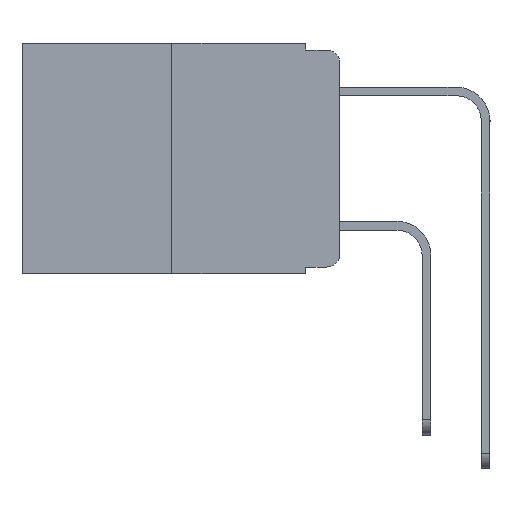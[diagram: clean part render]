
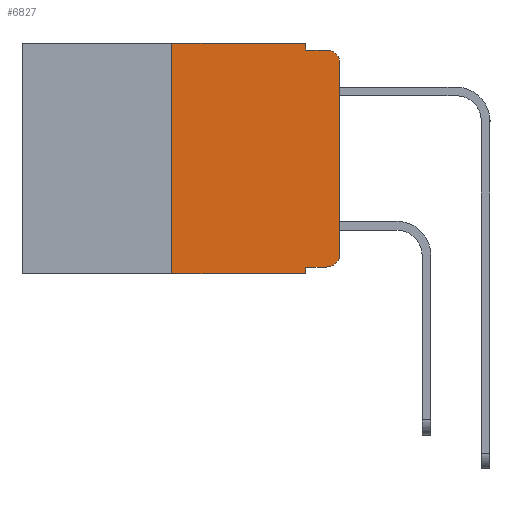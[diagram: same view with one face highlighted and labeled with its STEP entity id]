
A CAD part, left-side view. The second image highlights one B-rep face of the part: STEP entity #6827.
In plain terms, the highlighted planar face has unit normal (-1, 0, 0).
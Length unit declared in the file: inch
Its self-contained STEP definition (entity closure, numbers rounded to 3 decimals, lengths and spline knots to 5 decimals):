
#194 = ORIENTED_EDGE ( 'NONE', *, *, #5802, .T. ) ;
#305 = ORIENTED_EDGE ( 'NONE', *, *, #12336, .F. ) ;
#312 = PLANE ( 'NONE',  #7503 ) ;
#669 = LINE ( 'NONE', #23085, #15810 ) ;
#783 = VECTOR ( 'NONE', #23891, 39.37008 ) ;
#924 = ORIENTED_EDGE ( 'NONE', *, *, #17649, .T. ) ;
#1150 = EDGE_CURVE ( 'NONE', #8690, #19182, #22204, .T. ) ;
#1744 = CARTESIAN_POINT ( 'NONE',  ( 0., 0.051, 0. ) ) ;
#2332 = CARTESIAN_POINT ( 'NONE',  ( 0., 0., -0.313 ) ) ;
#2387 = ORIENTED_EDGE ( 'NONE', *, *, #1150, .F. ) ;
#2409 = VERTEX_POINT ( 'NONE', #2792 ) ;
#2776 = ORIENTED_EDGE ( 'NONE', *, *, #11029, .F. ) ;
#2792 = CARTESIAN_POINT ( 'NONE',  ( 0., 0.051, -0.01 ) ) ;
#3441 = DIRECTION ( 'NONE',  ( -1., 0., 0. ) ) ;
#3478 = DIRECTION ( 'NONE',  ( 0., 0., -1. ) ) ;
#3485 = EDGE_CURVE ( 'NONE', #17814, #13429, #20283, .T. ) ;
#3825 = ORIENTED_EDGE ( 'NONE', *, *, #8395, .F. ) ;
#4026 = CARTESIAN_POINT ( 'NONE',  ( 0., 0.02, -0.333 ) ) ;
#4243 = VERTEX_POINT ( 'NONE', #4026 ) ;
#4704 = CARTESIAN_POINT ( 'NONE',  ( 0., 0.051, -0.343 ) ) ;
#5216 = CARTESIAN_POINT ( 'NONE',  ( 0., 0.02, -0.313 ) ) ;
#5350 = CARTESIAN_POINT ( 'NONE',  ( 0., 0.051, 0. ) ) ;
#5802 = EDGE_CURVE ( 'NONE', #4243, #10560, #9116, .T. ) ;
#6376 = FACE_OUTER_BOUND ( 'NONE', #19559, .T. ) ;
#6600 = VECTOR ( 'NONE', #23822, 39.37008 ) ;
#6827 = ADVANCED_FACE ( 'NONE', ( #6376 ), #312, .F. ) ;
#7114 = EDGE_CURVE ( 'NONE', #15559, #4243, #21062, .T. ) ;
#7503 = AXIS2_PLACEMENT_3D ( 'NONE', #17648, #24567, #24156 ) ;
#7657 = CIRCLE ( 'NONE', #21750, 0.02 ) ;
#7786 = ORIENTED_EDGE ( 'NONE', *, *, #7114, .T. ) ;
#8268 = CARTESIAN_POINT ( 'NONE',  ( 0., 0.051, -0.01 ) ) ;
#8365 = CARTESIAN_POINT ( 'NONE',  ( 0., 0.02, -0.03 ) ) ;
#8395 = EDGE_CURVE ( 'NONE', #15559, #13429, #669, .T. ) ;
#8479 = DIRECTION ( 'NONE',  ( 0., -1., 0. ) ) ;
#8690 = VERTEX_POINT ( 'NONE', #20181 ) ;
#9111 = CARTESIAN_POINT ( 'NONE',  ( 0., 0.473, -0.343 ) ) ;
#9116 = CIRCLE ( 'NONE', #22555, 0.02 ) ;
#9568 = ORIENTED_EDGE ( 'NONE', *, *, #15020, .F. ) ;
#9575 = LINE ( 'NONE', #5350, #14199 ) ;
#9639 = VECTOR ( 'NONE', #15490, 39.37008 ) ;
#9720 = ORIENTED_EDGE ( 'NONE', *, *, #16343, .T. ) ;
#9856 = VECTOR ( 'NONE', #8479, 39.37008 ) ;
#10327 = DIRECTION ( 'NONE',  ( 0., 0., -1. ) ) ;
#10560 = VERTEX_POINT ( 'NONE', #2332 ) ;
#11029 = EDGE_CURVE ( 'NONE', #17814, #8690, #25164, .T. ) ;
#11262 = LINE ( 'NONE', #8268, #783 ) ;
#12336 = EDGE_CURVE ( 'NONE', #19182, #2409, #9575, .T. ) ;
#12668 = CARTESIAN_POINT ( 'NONE',  ( 0., 0.051, -0.333 ) ) ;
#13429 = VERTEX_POINT ( 'NONE', #4704 ) ;
#13446 = CARTESIAN_POINT ( 'NONE',  ( 0., 0.473, 0. ) ) ;
#13503 = CARTESIAN_POINT ( 'NONE',  ( 0., 0.25, 0. ) ) ;
#14199 = VECTOR ( 'NONE', #17154, 39.37008 ) ;
#14654 = LINE ( 'NONE', #18446, #23168 ) ;
#15020 = EDGE_CURVE ( 'NONE', #2409, #17962, #11262, .T. ) ;
#15097 = CARTESIAN_POINT ( 'NONE',  ( 0., 0.25, -0.343 ) ) ;
#15490 = DIRECTION ( 'NONE',  ( 0., 0., 1. ) ) ;
#15559 = VERTEX_POINT ( 'NONE', #21690 ) ;
#15810 = VECTOR ( 'NONE', #24978, 39.37008 ) ;
#16309 = CARTESIAN_POINT ( 'NONE',  ( 0., 0., -0.03 ) ) ;
#16343 = EDGE_CURVE ( 'NONE', #16357, #17962, #7657, .T. ) ;
#16357 = VERTEX_POINT ( 'NONE', #16309 ) ;
#17154 = DIRECTION ( 'NONE',  ( 0., 0., -1. ) ) ;
#17648 = CARTESIAN_POINT ( 'NONE',  ( 0., 0.473, 0. ) ) ;
#17649 = EDGE_CURVE ( 'NONE', #10560, #16357, #14654, .T. ) ;
#17814 = VERTEX_POINT ( 'NONE', #15097 ) ;
#17962 = VERTEX_POINT ( 'NONE', #25201 ) ;
#18446 = CARTESIAN_POINT ( 'NONE',  ( 0., 0., 0. ) ) ;
#19182 = VERTEX_POINT ( 'NONE', #1744 ) ;
#19559 = EDGE_LOOP ( 'NONE', ( #924, #9720, #9568, #305, #2387, #2776, #22140, #3825, #7786, #194 ) ) ;
#20181 = CARTESIAN_POINT ( 'NONE',  ( 0., 0.25, 0. ) ) ;
#20283 = LINE ( 'NONE', #9111, #9856 ) ;
#21062 = LINE ( 'NONE', #12668, #24932 ) ;
#21690 = CARTESIAN_POINT ( 'NONE',  ( 0., 0.051, -0.333 ) ) ;
#21750 = AXIS2_PLACEMENT_3D ( 'NONE', #8365, #22074, #10327 ) ;
#22074 = DIRECTION ( 'NONE',  ( -1., 0., 0. ) ) ;
#22140 = ORIENTED_EDGE ( 'NONE', *, *, #3485, .T. ) ;
#22204 = LINE ( 'NONE', #13446, #6600 ) ;
#22340 = DIRECTION ( 'NONE',  ( 0., 0., 1. ) ) ;
#22555 = AXIS2_PLACEMENT_3D ( 'NONE', #5216, #3441, #3478 ) ;
#23085 = CARTESIAN_POINT ( 'NONE',  ( 0., 0.051, 0. ) ) ;
#23168 = VECTOR ( 'NONE', #22340, 39.37008 ) ;
#23756 = DIRECTION ( 'NONE',  ( 0., -1., 0. ) ) ;
#23822 = DIRECTION ( 'NONE',  ( 0., -1., 0. ) ) ;
#23891 = DIRECTION ( 'NONE',  ( 0., -1., 0. ) ) ;
#24156 = DIRECTION ( 'NONE',  ( 0., 0., -1. ) ) ;
#24567 = DIRECTION ( 'NONE',  ( 1., 0., 0. ) ) ;
#24932 = VECTOR ( 'NONE', #23756, 39.37008 ) ;
#24978 = DIRECTION ( 'NONE',  ( 0., 0., -1. ) ) ;
#25164 = LINE ( 'NONE', #13503, #9639 ) ;
#25201 = CARTESIAN_POINT ( 'NONE',  ( 0., 0.02, -0.01 ) ) ;
